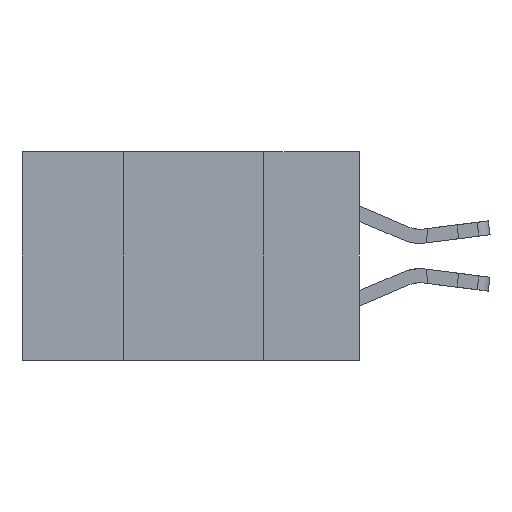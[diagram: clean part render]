
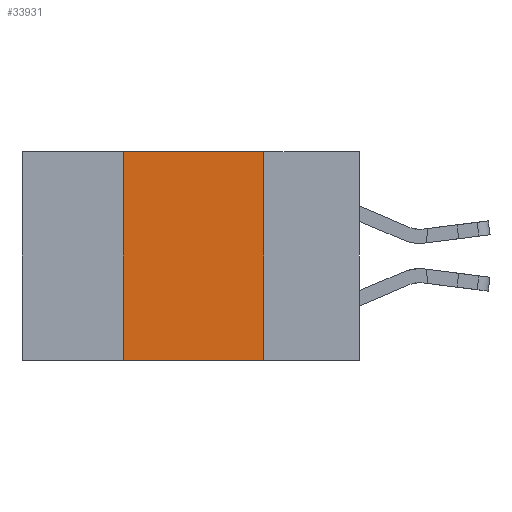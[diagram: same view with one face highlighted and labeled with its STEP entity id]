
A CAD part, left-side view. The second image highlights one B-rep face of the part: STEP entity #33931.
In plain terms, the highlighted planar face has unit normal (-1, 0, 0).
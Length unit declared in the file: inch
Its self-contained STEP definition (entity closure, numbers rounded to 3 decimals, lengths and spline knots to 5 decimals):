
#1364 = LINE ( 'NONE', #22395, #11927 ) ;
#1850 = LINE ( 'NONE', #22702, #33275 ) ;
#5085 = CARTESIAN_POINT ( 'NONE',  ( 0., 0.17, 0. ) ) ;
#6821 = LINE ( 'NONE', #33545, #27152 ) ;
#8089 = DIRECTION ( 'NONE',  ( 0., 0., -1. ) ) ;
#9064 = DIRECTION ( 'NONE',  ( 0., -1., 0. ) ) ;
#11196 = CARTESIAN_POINT ( 'NONE',  ( 0., 0.17, -0.37 ) ) ;
#11283 = VERTEX_POINT ( 'NONE', #11196 ) ;
#11927 = VECTOR ( 'NONE', #9064, 39.37008 ) ;
#13272 = EDGE_CURVE ( 'NONE', #29825, #11283, #1364, .T. ) ;
#13482 = ORIENTED_EDGE ( 'NONE', *, *, #22263, .F. ) ;
#14700 = DIRECTION ( 'NONE',  ( 0., -1., 0. ) ) ;
#18210 = EDGE_CURVE ( 'NONE', #26192, #27816, #6821, .T. ) ;
#18424 = ORIENTED_EDGE ( 'NONE', *, *, #18210, .F. ) ;
#18574 = VECTOR ( 'NONE', #31808, 39.37008 ) ;
#19241 = ORIENTED_EDGE ( 'NONE', *, *, #31335, .F. ) ;
#21196 = LINE ( 'NONE', #5085, #18574 ) ;
#21531 = CARTESIAN_POINT ( 'NONE',  ( 0., 0.17, 0. ) ) ;
#22263 = EDGE_CURVE ( 'NONE', #29825, #26192, #1850, .T. ) ;
#22395 = CARTESIAN_POINT ( 'NONE',  ( 0., 0.6, -0.37 ) ) ;
#22702 = CARTESIAN_POINT ( 'NONE',  ( 0., 0.42, 0. ) ) ;
#23017 = CARTESIAN_POINT ( 'NONE',  ( 0., 0.6, 0. ) ) ;
#23970 = CARTESIAN_POINT ( 'NONE',  ( 0., 0.42, 0. ) ) ;
#23971 = ORIENTED_EDGE ( 'NONE', *, *, #13272, .T. ) ;
#25226 = EDGE_LOOP ( 'NONE', ( #19241, #18424, #13482, #23971 ) ) ;
#26130 = DIRECTION ( 'NONE',  ( 1., 0., 0. ) ) ;
#26159 = CARTESIAN_POINT ( 'NONE',  ( 0., 0.42, -0.37 ) ) ;
#26192 = VERTEX_POINT ( 'NONE', #23970 ) ;
#27152 = VECTOR ( 'NONE', #14700, 39.37008 ) ;
#27816 = VERTEX_POINT ( 'NONE', #21531 ) ;
#28733 = PLANE ( 'NONE',  #33277 ) ;
#29825 = VERTEX_POINT ( 'NONE', #26159 ) ;
#31335 = EDGE_CURVE ( 'NONE', #27816, #11283, #21196, .T. ) ;
#31354 = FACE_OUTER_BOUND ( 'NONE', #25226, .T. ) ;
#31808 = DIRECTION ( 'NONE',  ( 0., 0., -1. ) ) ;
#33275 = VECTOR ( 'NONE', #33311, 39.37008 ) ;
#33277 = AXIS2_PLACEMENT_3D ( 'NONE', #23017, #26130, #8089 ) ;
#33311 = DIRECTION ( 'NONE',  ( 0., 0., 1. ) ) ;
#33545 = CARTESIAN_POINT ( 'NONE',  ( 0., 0.6, 0. ) ) ;
#33931 = ADVANCED_FACE ( 'NONE', ( #31354 ), #28733, .F. ) ;
